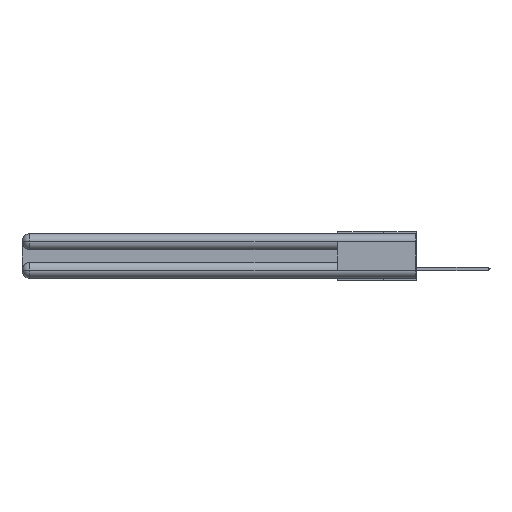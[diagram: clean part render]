
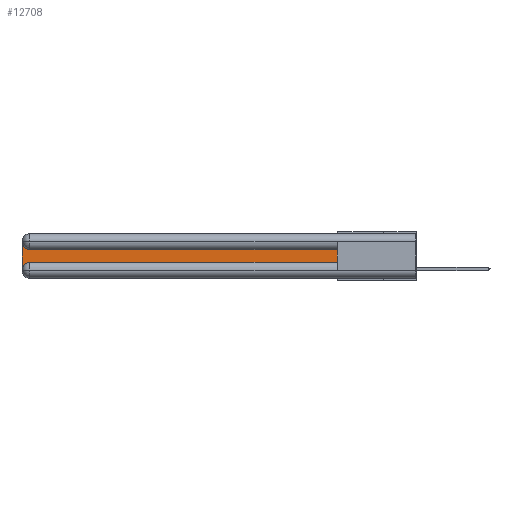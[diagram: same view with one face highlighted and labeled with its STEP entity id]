
A CAD part, left-side view. The second image highlights one B-rep face of the part: STEP entity #12708.
In plain terms, the highlighted planar face has unit normal (-1, 0, 0).
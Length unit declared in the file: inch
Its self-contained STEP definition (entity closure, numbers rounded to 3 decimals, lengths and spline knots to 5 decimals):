
#1625 = VECTOR ( 'NONE', #21684, 39.37008 ) ;
#3239 = ORIENTED_EDGE ( 'NONE', *, *, #26491, .T. ) ;
#3278 = AXIS2_PLACEMENT_3D ( 'NONE', #17501, #27791, #12015 ) ;
#3382 = CARTESIAN_POINT ( 'NONE',  ( 0.075, 0.6, -0.1225 ) ) ;
#4149 = CARTESIAN_POINT ( 'NONE',  ( 0.075, 3., -0.2175 ) ) ;
#4296 = DIRECTION ( 'NONE',  ( 1., 0., 0. ) ) ;
#5832 = EDGE_LOOP ( 'NONE', ( #23256, #29143, #23464, #3239, #17688, #10327 ) ) ;
#7252 = CARTESIAN_POINT ( 'NONE',  ( 0.075, 0.6, -0.2175 ) ) ;
#7879 = CARTESIAN_POINT ( 'NONE',  ( 0.075, 2.94, -0.2175 ) ) ;
#7978 = CARTESIAN_POINT ( 'NONE',  ( 0.075, 0.6, -0.2175 ) ) ;
#8283 = VERTEX_POINT ( 'NONE', #7879 ) ;
#8714 = LINE ( 'NONE', #3382, #1625 ) ;
#9182 = PLANE ( 'NONE',  #3278 ) ;
#10090 = EDGE_CURVE ( 'NONE', #19696, #13897, #17219, .T. ) ;
#10173 = CARTESIAN_POINT ( 'NONE',  ( 0.075, 2.94, -0.2775 ) ) ;
#10327 = ORIENTED_EDGE ( 'NONE', *, *, #31300, .T. ) ;
#11177 = CARTESIAN_POINT ( 'NONE',  ( 0.075, 3., -0.0625 ) ) ;
#11712 = EDGE_CURVE ( 'NONE', #29000, #19696, #8714, .T. ) ;
#11754 = CARTESIAN_POINT ( 'NONE',  ( 0.075, 3., -0.2775 ) ) ;
#12015 = DIRECTION ( 'NONE',  ( 0., 0., -1. ) ) ;
#12708 = ADVANCED_FACE ( 'NONE', ( #24848 ), #9182, .F. ) ;
#12821 = DIRECTION ( 'NONE',  ( 0., 0., -1. ) ) ;
#12834 = AXIS2_PLACEMENT_3D ( 'NONE', #33729, #4296, #12821 ) ;
#13897 = VERTEX_POINT ( 'NONE', #11177 ) ;
#14532 = CARTESIAN_POINT ( 'NONE',  ( 0.075, 2.94, -0.1225 ) ) ;
#15304 = EDGE_CURVE ( 'NONE', #8283, #23437, #27712, .T. ) ;
#16951 = VECTOR ( 'NONE', #27903, 39.37008 ) ;
#17219 = CIRCLE ( 'NONE', #12834, 0.06 ) ;
#17222 = VERTEX_POINT ( 'NONE', #11754 ) ;
#17501 = CARTESIAN_POINT ( 'NONE',  ( 0.075, 3., -0.1225 ) ) ;
#17688 = ORIENTED_EDGE ( 'NONE', *, *, #15304, .T. ) ;
#18986 = LINE ( 'NONE', #25238, #16951 ) ;
#19037 = VECTOR ( 'NONE', #27772, 39.37008 ) ;
#19632 = AXIS2_PLACEMENT_3D ( 'NONE', #10173, #20900, #28784 ) ;
#19696 = VERTEX_POINT ( 'NONE', #14532 ) ;
#20900 = DIRECTION ( 'NONE',  ( 1., 0., 0. ) ) ;
#21684 = DIRECTION ( 'NONE',  ( 0., 1., 0. ) ) ;
#21732 = DIRECTION ( 'NONE',  ( 0., -1., 0. ) ) ;
#22764 = VECTOR ( 'NONE', #21732, 39.37008 ) ;
#22990 = EDGE_CURVE ( 'NONE', #13897, #17222, #33974, .T. ) ;
#23256 = ORIENTED_EDGE ( 'NONE', *, *, #11712, .T. ) ;
#23437 = VERTEX_POINT ( 'NONE', #7252 ) ;
#23464 = ORIENTED_EDGE ( 'NONE', *, *, #22990, .T. ) ;
#24848 = FACE_OUTER_BOUND ( 'NONE', #5832, .T. ) ;
#25238 = CARTESIAN_POINT ( 'NONE',  ( 0.075, 0.6, -0.2175 ) ) ;
#26491 = EDGE_CURVE ( 'NONE', #17222, #8283, #29242, .T. ) ;
#27712 = LINE ( 'NONE', #7978, #22764 ) ;
#27772 = DIRECTION ( 'NONE',  ( 0., 0., -1. ) ) ;
#27791 = DIRECTION ( 'NONE',  ( 1., 0., 0. ) ) ;
#27903 = DIRECTION ( 'NONE',  ( 0., 0., 1. ) ) ;
#28784 = DIRECTION ( 'NONE',  ( 0., 0., -1. ) ) ;
#29000 = VERTEX_POINT ( 'NONE', #30036 ) ;
#29143 = ORIENTED_EDGE ( 'NONE', *, *, #10090, .T. ) ;
#29242 = CIRCLE ( 'NONE', #19632, 0.06 ) ;
#30036 = CARTESIAN_POINT ( 'NONE',  ( 0.075, 0.6, -0.1225 ) ) ;
#31300 = EDGE_CURVE ( 'NONE', #23437, #29000, #18986, .T. ) ;
#33729 = CARTESIAN_POINT ( 'NONE',  ( 0.075, 2.94, -0.0625 ) ) ;
#33974 = LINE ( 'NONE', #4149, #19037 ) ;
